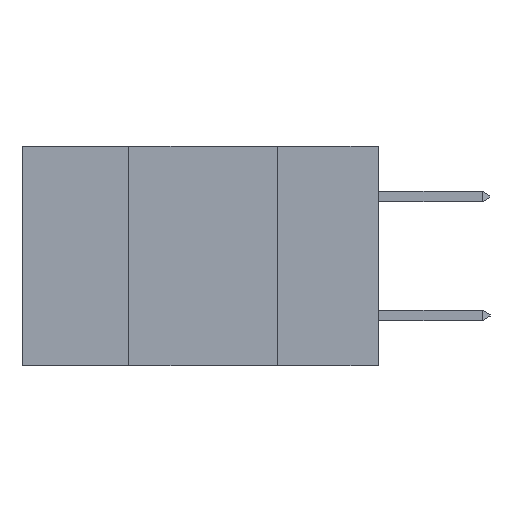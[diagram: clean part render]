
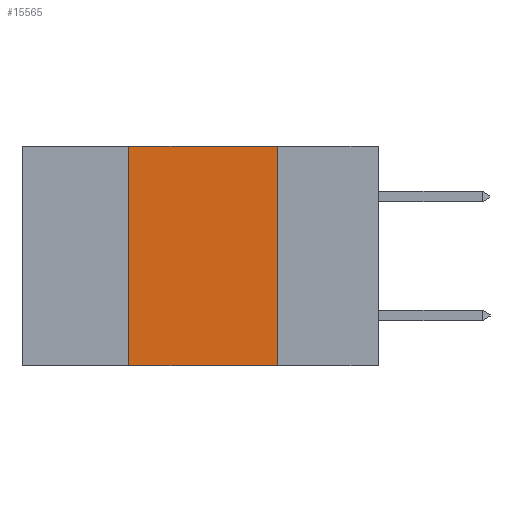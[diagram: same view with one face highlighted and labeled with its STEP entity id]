
A CAD part, left-side view. The second image highlights one B-rep face of the part: STEP entity #15565.
In plain terms, the highlighted planar face has unit normal (-1, 0, 0).
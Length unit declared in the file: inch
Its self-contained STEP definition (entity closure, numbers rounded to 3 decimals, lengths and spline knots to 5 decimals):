
#231 = CARTESIAN_POINT ( 'NONE',  ( 0., 0.17, -0.37 ) ) ;
#1371 = FACE_OUTER_BOUND ( 'NONE', #5066, .T. ) ;
#2870 = VECTOR ( 'NONE', #15452, 39.37008 ) ;
#2937 = CARTESIAN_POINT ( 'NONE',  ( 0., 0.6, -0.37 ) ) ;
#3128 = CARTESIAN_POINT ( 'NONE',  ( 0., 0.17, 0. ) ) ;
#4515 = VERTEX_POINT ( 'NONE', #23924 ) ;
#5066 = EDGE_LOOP ( 'NONE', ( #14869, #25015, #7118, #18187 ) ) ;
#5075 = CARTESIAN_POINT ( 'NONE',  ( 0., 0.42, 0. ) ) ;
#7118 = ORIENTED_EDGE ( 'NONE', *, *, #19435, .F. ) ;
#8334 = EDGE_CURVE ( 'NONE', #4515, #15836, #20003, .T. ) ;
#8340 = CARTESIAN_POINT ( 'NONE',  ( 0., 0.42, -0.37 ) ) ;
#9318 = EDGE_CURVE ( 'NONE', #21599, #23684, #23911, .T. ) ;
#9478 = VECTOR ( 'NONE', #11619, 39.37008 ) ;
#11429 = DIRECTION ( 'NONE',  ( 1., 0., 0. ) ) ;
#11619 = DIRECTION ( 'NONE',  ( 0., -1., 0. ) ) ;
#12245 = DIRECTION ( 'NONE',  ( 0., 0., -1. ) ) ;
#12463 = LINE ( 'NONE', #231, #17124 ) ;
#14869 = ORIENTED_EDGE ( 'NONE', *, *, #22207, .F. ) ;
#15452 = DIRECTION ( 'NONE',  ( 0., -1., 0. ) ) ;
#15533 = VECTOR ( 'NONE', #24115, 39.37008 ) ;
#15565 = ADVANCED_FACE ( 'NONE', ( #1371 ), #23237, .F. ) ;
#15836 = VERTEX_POINT ( 'NONE', #20267 ) ;
#17084 = CARTESIAN_POINT ( 'NONE',  ( 0., 0.6, 0. ) ) ;
#17124 = VECTOR ( 'NONE', #12245, 39.37008 ) ;
#18187 = ORIENTED_EDGE ( 'NONE', *, *, #8334, .T. ) ;
#18427 = AXIS2_PLACEMENT_3D ( 'NONE', #25132, #11429, #25226 ) ;
#19435 = EDGE_CURVE ( 'NONE', #4515, #21599, #25745, .T. ) ;
#20003 = LINE ( 'NONE', #2937, #9478 ) ;
#20267 = CARTESIAN_POINT ( 'NONE',  ( 0., 0.17, -0.37 ) ) ;
#21599 = VERTEX_POINT ( 'NONE', #5075 ) ;
#22207 = EDGE_CURVE ( 'NONE', #23684, #15836, #12463, .T. ) ;
#23237 = PLANE ( 'NONE',  #18427 ) ;
#23684 = VERTEX_POINT ( 'NONE', #3128 ) ;
#23911 = LINE ( 'NONE', #17084, #2870 ) ;
#23924 = CARTESIAN_POINT ( 'NONE',  ( 0., 0.42, -0.37 ) ) ;
#24115 = DIRECTION ( 'NONE',  ( 0., 0., 1. ) ) ;
#25015 = ORIENTED_EDGE ( 'NONE', *, *, #9318, .F. ) ;
#25132 = CARTESIAN_POINT ( 'NONE',  ( 0., 0.6, 0. ) ) ;
#25226 = DIRECTION ( 'NONE',  ( 0., 0., -1. ) ) ;
#25745 = LINE ( 'NONE', #8340, #15533 ) ;
